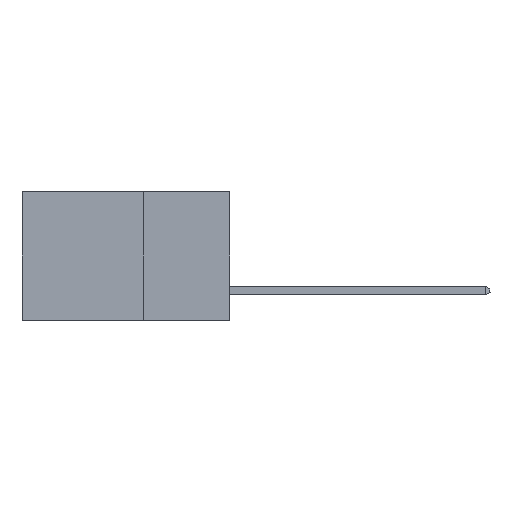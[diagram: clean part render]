
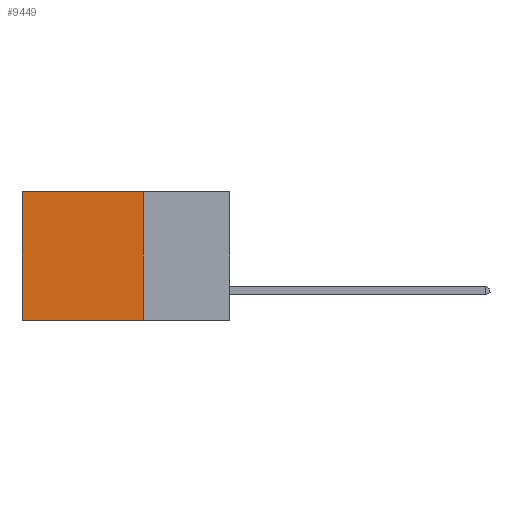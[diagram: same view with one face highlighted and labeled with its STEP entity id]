
A CAD part, left-side view. The second image highlights one B-rep face of the part: STEP entity #9449.
In plain terms, the highlighted planar face has unit normal (-1, 0, 0).
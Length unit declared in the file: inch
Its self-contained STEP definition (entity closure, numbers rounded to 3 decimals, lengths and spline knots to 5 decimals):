
#86 = CARTESIAN_POINT ( 'NONE',  ( 0.298, 0.25, 0. ) ) ;
#385 = CARTESIAN_POINT ( 'NONE',  ( 0.298, 0.25, 0. ) ) ;
#576 = CARTESIAN_POINT ( 'NONE',  ( 0.298, 0.25, -0.37 ) ) ;
#1024 = ORIENTED_EDGE ( 'NONE', *, *, #4143, .F. ) ;
#1059 = VECTOR ( 'NONE', #2021, 39.37008 ) ;
#1433 = VECTOR ( 'NONE', #8537, 39.37008 ) ;
#1880 = LINE ( 'NONE', #4870, #10185 ) ;
#2021 = DIRECTION ( 'NONE',  ( 0., 1., 0. ) ) ;
#2196 = LINE ( 'NONE', #576, #9605 ) ;
#3259 = ORIENTED_EDGE ( 'NONE', *, *, #7385, .T. ) ;
#3403 = ORIENTED_EDGE ( 'NONE', *, *, #4123, .F. ) ;
#3681 = CARTESIAN_POINT ( 'NONE',  ( 0.298, 0.6, -0.37 ) ) ;
#3689 = ORIENTED_EDGE ( 'NONE', *, *, #9985, .T. ) ;
#4123 = EDGE_CURVE ( 'NONE', #8897, #4694, #2196, .T. ) ;
#4143 = EDGE_CURVE ( 'NONE', #5419, #8897, #8253, .T. ) ;
#4694 = VERTEX_POINT ( 'NONE', #3681 ) ;
#4870 = CARTESIAN_POINT ( 'NONE',  ( 0.298, 0.6, 0. ) ) ;
#5023 = PLANE ( 'NONE',  #10280 ) ;
#5419 = VERTEX_POINT ( 'NONE', #10937 ) ;
#6316 = CARTESIAN_POINT ( 'NONE',  ( 0.298, 0.6, 0. ) ) ;
#6566 = DIRECTION ( 'NONE',  ( 0., 1., 0. ) ) ;
#6786 = VERTEX_POINT ( 'NONE', #6316 ) ;
#6918 = LINE ( 'NONE', #385, #1059 ) ;
#6983 = DIRECTION ( 'NONE',  ( 1., 0., 0. ) ) ;
#7385 = EDGE_CURVE ( 'NONE', #5419, #6786, #6918, .T. ) ;
#7998 = DIRECTION ( 'NONE',  ( 0., 0., -1. ) ) ;
#8253 = LINE ( 'NONE', #10423, #1433 ) ;
#8537 = DIRECTION ( 'NONE',  ( 0., 0., -1. ) ) ;
#8897 = VERTEX_POINT ( 'NONE', #11109 ) ;
#9029 = EDGE_LOOP ( 'NONE', ( #3689, #3403, #1024, #3259 ) ) ;
#9449 = ADVANCED_FACE ( 'NONE', ( #10828 ), #5023, .F. ) ;
#9605 = VECTOR ( 'NONE', #6566, 39.37008 ) ;
#9985 = EDGE_CURVE ( 'NONE', #6786, #4694, #1880, .T. ) ;
#10185 = VECTOR ( 'NONE', #11746, 39.37008 ) ;
#10280 = AXIS2_PLACEMENT_3D ( 'NONE', #86, #6983, #7998 ) ;
#10423 = CARTESIAN_POINT ( 'NONE',  ( 0.298, 0.25, 0. ) ) ;
#10828 = FACE_OUTER_BOUND ( 'NONE', #9029, .T. ) ;
#10937 = CARTESIAN_POINT ( 'NONE',  ( 0.298, 0.25, 0. ) ) ;
#11109 = CARTESIAN_POINT ( 'NONE',  ( 0.298, 0.25, -0.37 ) ) ;
#11746 = DIRECTION ( 'NONE',  ( 0., 0., -1. ) ) ;
